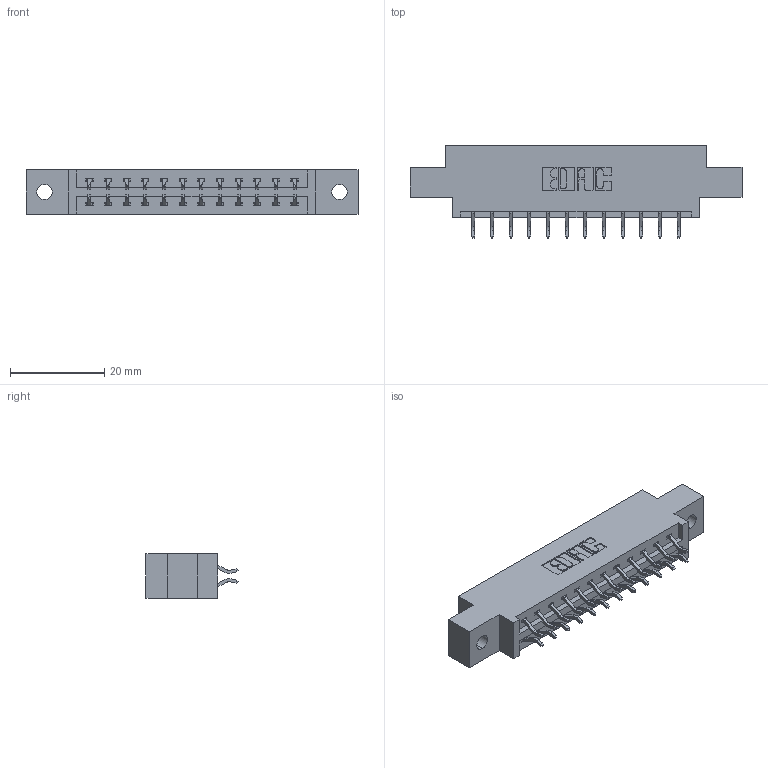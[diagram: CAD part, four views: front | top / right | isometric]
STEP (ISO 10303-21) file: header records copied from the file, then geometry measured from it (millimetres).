
FILE_DESCRIPTION (( 'STEP AP203' ), '1' );
FILE_NAME ('337-024-556-802.STEP', '2018-08-06T01:42:28', ( '' ), ( '' ), 'SwSTEP 2.0', 'SolidWorks 2016', '' );
FILE_SCHEMA (( 'CONFIG_CONTROL_DESIGN' ));
Length unit declared in the file: inch
Products named in the file (3): 337 Part_0.170 Offset - 0.128 Dia; 345-292-001_556 Tail; 337-024-556-802
Assembly tree (25 placements, depth 2):
  337-024-556-802
    337 Part_0.170 Offset - 0.128 Dia
    345-292-001_556 Tail  x24
Bounding box: 70.56 x 19.57 x 9.4 mm (x, y, z)
Volume: 6881.8 mm3; surface area: 7298.3 mm2
Topology: 25 solids, 25 shells, 1558 faces, 4619 edges, 3046 vertices
Faces by surface type: plane 1082, cylinder 476
Entity records: 13539 total; most frequent: CARTESIAN_POINT 2322, ORIENTED_EDGE 2246, DIRECTION 2019, EDGE_CURVE 1123, LINE 987, VECTOR 987, VERTEX_POINT 746, AXIS2_PLACEMENT_3D 516
